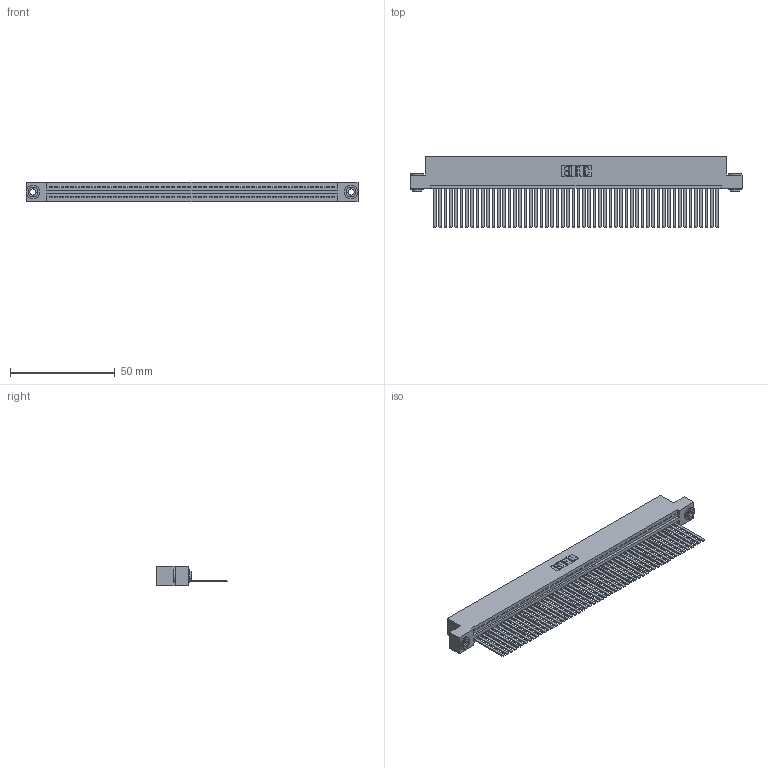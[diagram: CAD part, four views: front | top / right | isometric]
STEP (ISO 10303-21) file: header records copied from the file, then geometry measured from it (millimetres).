
FILE_DESCRIPTION (( 'STEP AP203' ), '1' );
FILE_NAME ('345-054-544-103.STEP', '2018-09-23T23:56:27', ( '' ), ( '' ), 'SwSTEP 2.0', 'SolidWorks 2016', '' );
FILE_SCHEMA (( 'CONFIG_CONTROL_DESIGN' ));
Length unit declared in the file: inch
Products named in the file (4): 345-250-002_345-250-002-102; 345-054-544-103; 345 Part_Flush Mounting Lugs - 0.156 Dia-TH; 345-292-001_345-293-144
Assembly tree (57 placements, depth 2):
  345-054-544-103
    345 Part_Flush Mounting Lugs - 0.156 Dia-TH
    345-292-001_345-293-144  x54
    345-250-002_345-250-002-102  x2
Bounding box: 158.37 x 33.96 x 9.4 mm (x, y, z)
Volume: 15785.1 mm3; surface area: 23232.1 mm2
Topology: 57 solids, 57 shells, 2972 faces, 8949 edges, 5890 vertices
Faces by surface type: plane 2034, cylinder 930, cone 8
Entity records: 39492 total; most frequent: CARTESIAN_POINT 6817, ORIENTED_EDGE 6798, DIRECTION 5965, EDGE_CURVE 3399, LINE 3031, VECTOR 3031, VERTEX_POINT 2262, AXIS2_PLACEMENT_3D 1467
